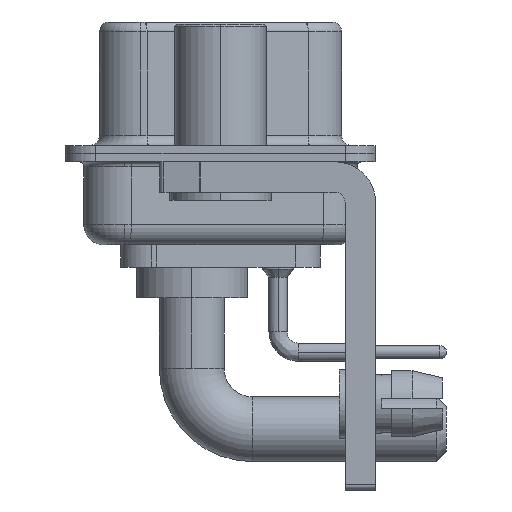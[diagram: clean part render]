
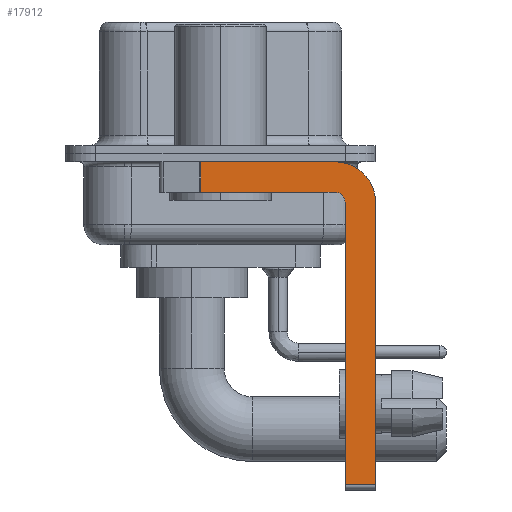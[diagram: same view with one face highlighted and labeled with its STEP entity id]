
A CAD part, left-side view. The second image highlights one B-rep face of the part: STEP entity #17912.
In plain terms, the highlighted planar face has unit normal (-1, 0, 0).
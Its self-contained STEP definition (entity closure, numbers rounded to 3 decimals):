
#137 = EDGE_CURVE ( 'NONE', #1641, #4801, #19414, .T. ) ;
#139 = CARTESIAN_POINT ( 'NONE',  ( -2.9, 0.978, -1.9 ) ) ;
#216 = CARTESIAN_POINT ( 'NONE',  ( -2.9, -5.65, -2.4 ) ) ;
#764 = CARTESIAN_POINT ( 'NONE',  ( -2.9, -7.65, -2.4 ) ) ;
#812 = VERTEX_POINT ( 'NONE', #24254 ) ;
#1022 = LINE ( 'NONE', #20563, #24357 ) ;
#1121 = ORIENTED_EDGE ( 'NONE', *, *, #8672, .F. ) ;
#1211 = VECTOR ( 'NONE', #3147, 1000. ) ;
#1307 = VERTEX_POINT ( 'NONE', #23807 ) ;
#1495 = EDGE_LOOP ( 'NONE', ( #15271, #5652, #25417, #4425, #24068, #11512, #8944, #1121 ) ) ;
#1641 = VERTEX_POINT ( 'NONE', #25853 ) ;
#1658 = VECTOR ( 'NONE', #17315, 1000. ) ;
#2140 = CARTESIAN_POINT ( 'NONE',  ( -2.9, -5.65, -2.4 ) ) ;
#2961 = CARTESIAN_POINT ( 'NONE',  ( -2.9, -6.15, -2.4 ) ) ;
#3147 = DIRECTION ( 'NONE',  ( 0., 1., 0. ) ) ;
#3333 = EDGE_CURVE ( 'NONE', #3802, #3695, #10194, .T. ) ;
#3695 = VERTEX_POINT ( 'NONE', #139 ) ;
#3802 = VERTEX_POINT ( 'NONE', #20922 ) ;
#3822 = DIRECTION ( 'NONE',  ( 1., 0., 0. ) ) ;
#4425 = ORIENTED_EDGE ( 'NONE', *, *, #5671, .F. ) ;
#4547 = EDGE_CURVE ( 'NONE', #1641, #1307, #1022, .T. ) ;
#4801 = VERTEX_POINT ( 'NONE', #2961 ) ;
#5652 = ORIENTED_EDGE ( 'NONE', *, *, #3333, .T. ) ;
#5671 = EDGE_CURVE ( 'NONE', #4801, #17592, #13875, .T. ) ;
#7319 = LINE ( 'NONE', #13256, #19644 ) ;
#8672 = EDGE_CURVE ( 'NONE', #26157, #812, #25451, .T. ) ;
#8944 = ORIENTED_EDGE ( 'NONE', *, *, #20184, .F. ) ;
#9076 = DIRECTION ( 'NONE',  ( 0., 0., -1. ) ) ;
#10194 = LINE ( 'NONE', #17324, #11004 ) ;
#10425 = EDGE_CURVE ( 'NONE', #3802, #26157, #7319, .T. ) ;
#10874 = DIRECTION ( 'NONE',  ( -1., 0., 0. ) ) ;
#11004 = VECTOR ( 'NONE', #18633, 1000. ) ;
#11512 = ORIENTED_EDGE ( 'NONE', *, *, #4547, .T. ) ;
#12142 = AXIS2_PLACEMENT_3D ( 'NONE', #14243, #24811, #26618 ) ;
#12249 = DIRECTION ( 'NONE',  ( 0., 0., -1. ) ) ;
#12571 = VECTOR ( 'NONE', #9076, 1000. ) ;
#13256 = CARTESIAN_POINT ( 'NONE',  ( -2.9, 3., -0.4 ) ) ;
#13655 = CARTESIAN_POINT ( 'NONE',  ( -2.9, -5.65, -1.9 ) ) ;
#13875 = CIRCLE ( 'NONE', #22752, 0.5 ) ;
#14070 = LINE ( 'NONE', #13655, #1211 ) ;
#14243 = CARTESIAN_POINT ( 'NONE',  ( -2.9, -5.65, -2.4 ) ) ;
#14709 = EDGE_CURVE ( 'NONE', #17592, #3695, #14070, .T. ) ;
#15271 = ORIENTED_EDGE ( 'NONE', *, *, #10425, .F. ) ;
#15829 = DIRECTION ( 'NONE',  ( 0., -1., 0. ) ) ;
#16925 = PLANE ( 'NONE',  #22228 ) ;
#17315 = DIRECTION ( 'NONE',  ( 0., 0., 1. ) ) ;
#17324 = CARTESIAN_POINT ( 'NONE',  ( -2.9, 0.978, -1.9 ) ) ;
#17592 = VERTEX_POINT ( 'NONE', #21967 ) ;
#17912 = ADVANCED_FACE ( 'NONE', ( #27377 ), #16925, .F. ) ;
#18633 = DIRECTION ( 'NONE',  ( 0., 0., -1. ) ) ;
#19414 = LINE ( 'NONE', #25678, #1658 ) ;
#19579 = CARTESIAN_POINT ( 'NONE',  ( -2.9, -5.65, -0.4 ) ) ;
#19644 = VECTOR ( 'NONE', #25919, 1000. ) ;
#20184 = EDGE_CURVE ( 'NONE', #812, #1307, #26286, .T. ) ;
#20563 = CARTESIAN_POINT ( 'NONE',  ( -2.9, -5.65, -16.35 ) ) ;
#20922 = CARTESIAN_POINT ( 'NONE',  ( -2.9, 0.978, -0.4 ) ) ;
#21967 = CARTESIAN_POINT ( 'NONE',  ( -2.9, -5.65, -1.9 ) ) ;
#22228 = AXIS2_PLACEMENT_3D ( 'NONE', #2140, #3822, #12249 ) ;
#22752 = AXIS2_PLACEMENT_3D ( 'NONE', #216, #10874, #22961 ) ;
#22961 = DIRECTION ( 'NONE',  ( 0., 0., 1. ) ) ;
#23807 = CARTESIAN_POINT ( 'NONE',  ( -2.9, -7.65, -16.35 ) ) ;
#24068 = ORIENTED_EDGE ( 'NONE', *, *, #137, .F. ) ;
#24254 = CARTESIAN_POINT ( 'NONE',  ( -2.9, -7.65, -2.4 ) ) ;
#24357 = VECTOR ( 'NONE', #15829, 1000. ) ;
#24811 = DIRECTION ( 'NONE',  ( 1., 0., 0. ) ) ;
#25417 = ORIENTED_EDGE ( 'NONE', *, *, #14709, .F. ) ;
#25451 = CIRCLE ( 'NONE', #12142, 2. ) ;
#25678 = CARTESIAN_POINT ( 'NONE',  ( -2.9, -6.15, -16.6 ) ) ;
#25853 = CARTESIAN_POINT ( 'NONE',  ( -2.9, -6.15, -16.35 ) ) ;
#25919 = DIRECTION ( 'NONE',  ( 0., -1., 0. ) ) ;
#26157 = VERTEX_POINT ( 'NONE', #19579 ) ;
#26286 = LINE ( 'NONE', #764, #12571 ) ;
#26618 = DIRECTION ( 'NONE',  ( 0., 0., -1. ) ) ;
#27377 = FACE_OUTER_BOUND ( 'NONE', #1495, .T. ) ;
